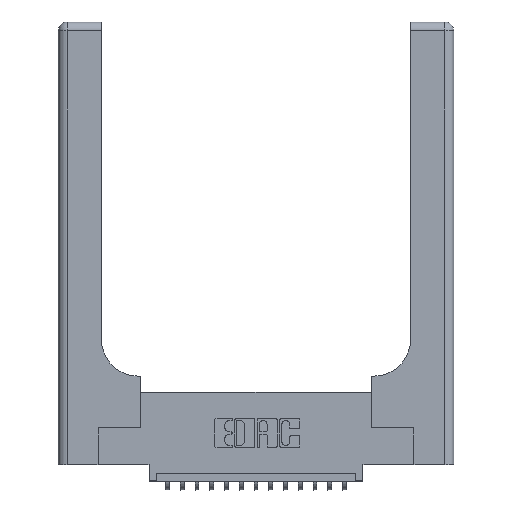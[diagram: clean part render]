
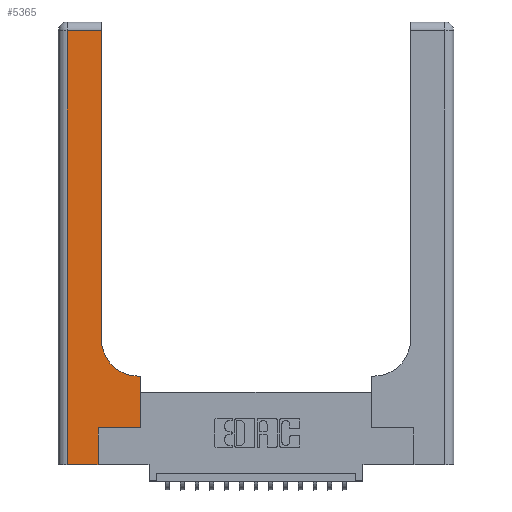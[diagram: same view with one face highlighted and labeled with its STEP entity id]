
A CAD part, top view. The second image highlights one B-rep face of the part: STEP entity #5365.
In plain terms, the highlighted planar face has unit normal (0, 0, 1).
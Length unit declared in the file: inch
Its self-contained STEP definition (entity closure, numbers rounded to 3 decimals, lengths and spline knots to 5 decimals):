
#322 = LINE ( 'NONE', #1450, #18718 ) ;
#375 = FACE_OUTER_BOUND ( 'NONE', #7149, .T. ) ;
#377 = CARTESIAN_POINT ( 'NONE',  ( 0.06, 2.94, 0.37 ) ) ;
#713 = CARTESIAN_POINT ( 'NONE',  ( 0., 2.94, 0.37 ) ) ;
#1450 = CARTESIAN_POINT ( 'NONE',  ( 0.5585, 0.25, 0.37 ) ) ;
#1487 = CARTESIAN_POINT ( 'NONE',  ( 0.5415, 0.85, 0.37 ) ) ;
#2405 = EDGE_CURVE ( 'NONE', #10606, #6755, #6256, .T. ) ;
#2713 = ORIENTED_EDGE ( 'NONE', *, *, #6560, .T. ) ;
#2805 = CARTESIAN_POINT ( 'NONE',  ( 0.269, 0.25, 0.37 ) ) ;
#3157 = CARTESIAN_POINT ( 'NONE',  ( 0.2915, 3., 0.37 ) ) ;
#3464 = CARTESIAN_POINT ( 'NONE',  ( 0.2915, 0.6, 0.37 ) ) ;
#3772 = EDGE_CURVE ( 'NONE', #4561, #6391, #17874, .T. ) ;
#3784 = ORIENTED_EDGE ( 'NONE', *, *, #3772, .T. ) ;
#4359 = CARTESIAN_POINT ( 'NONE',  ( 0., 0., 0.37 ) ) ;
#4384 = LINE ( 'NONE', #8307, #5082 ) ;
#4395 = AXIS2_PLACEMENT_3D ( 'NONE', #1487, #4442, #5828 ) ;
#4442 = DIRECTION ( 'NONE',  ( 0., 0., -1. ) ) ;
#4561 = VERTEX_POINT ( 'NONE', #8616 ) ;
#4680 = DIRECTION ( 'NONE',  ( 1., 0., 0. ) ) ;
#4895 = DIRECTION ( 'NONE',  ( 0., -1., 0. ) ) ;
#4956 = VERTEX_POINT ( 'NONE', #13395 ) ;
#5082 = VECTOR ( 'NONE', #11375, 39.37008 ) ;
#5114 = DIRECTION ( 'NONE',  ( -1., 0., 0. ) ) ;
#5365 = ADVANCED_FACE ( 'NONE', ( #375 ), #12111, .F. ) ;
#5442 = EDGE_CURVE ( 'NONE', #11132, #18178, #17842, .T. ) ;
#5612 = DIRECTION ( 'NONE',  ( 0., 1., 0. ) ) ;
#5828 = DIRECTION ( 'NONE',  ( 1., 0., 0. ) ) ;
#6236 = ORIENTED_EDGE ( 'NONE', *, *, #13190, .T. ) ;
#6256 = LINE ( 'NONE', #3464, #8334 ) ;
#6391 = VERTEX_POINT ( 'NONE', #9600 ) ;
#6426 = VECTOR ( 'NONE', #7838, 39.37008 ) ;
#6560 = EDGE_CURVE ( 'NONE', #4956, #10606, #322, .T. ) ;
#6755 = VERTEX_POINT ( 'NONE', #12718 ) ;
#7149 = EDGE_LOOP ( 'NONE', ( #3784, #6236, #11499, #14602, #11961, #16135, #2713, #11330, #9094 ) ) ;
#7528 = DIRECTION ( 'NONE',  ( -1., 0., 0. ) ) ;
#7838 = DIRECTION ( 'NONE',  ( 1., 0., 0. ) ) ;
#8307 = CARTESIAN_POINT ( 'NONE',  ( 0.269, 0., 0.37 ) ) ;
#8334 = VECTOR ( 'NONE', #16461, 39.37008 ) ;
#8616 = CARTESIAN_POINT ( 'NONE',  ( 0.2915, 0.85, 0.37 ) ) ;
#8687 = VECTOR ( 'NONE', #5114, 39.37008 ) ;
#8854 = EDGE_CURVE ( 'NONE', #6755, #4561, #9188, .T. ) ;
#8856 = CARTESIAN_POINT ( 'NONE',  ( 0.06, 0., 0.37 ) ) ;
#9094 = ORIENTED_EDGE ( 'NONE', *, *, #8854, .T. ) ;
#9162 = DIRECTION ( 'NONE',  ( 0., 0., -1. ) ) ;
#9188 = CIRCLE ( 'NONE', #4395, 0.25 ) ;
#9600 = CARTESIAN_POINT ( 'NONE',  ( 0.2915, 2.94, 0.37 ) ) ;
#10606 = VERTEX_POINT ( 'NONE', #16197 ) ;
#10868 = VERTEX_POINT ( 'NONE', #2805 ) ;
#11132 = VERTEX_POINT ( 'NONE', #377 ) ;
#11330 = ORIENTED_EDGE ( 'NONE', *, *, #2405, .T. ) ;
#11375 = DIRECTION ( 'NONE',  ( 0., 1., 0. ) ) ;
#11397 = EDGE_CURVE ( 'NONE', #17665, #10868, #4384, .T. ) ;
#11499 = ORIENTED_EDGE ( 'NONE', *, *, #5442, .T. ) ;
#11740 = DIRECTION ( 'NONE',  ( 0., 1., 0. ) ) ;
#11921 = EDGE_CURVE ( 'NONE', #10868, #4956, #14277, .T. ) ;
#11961 = ORIENTED_EDGE ( 'NONE', *, *, #11397, .T. ) ;
#11970 = CARTESIAN_POINT ( 'NONE',  ( 0., 3., 0.37 ) ) ;
#12111 = PLANE ( 'NONE',  #15451 ) ;
#12405 = LINE ( 'NONE', #4359, #18140 ) ;
#12718 = CARTESIAN_POINT ( 'NONE',  ( 0.5415, 0.6, 0.37 ) ) ;
#13190 = EDGE_CURVE ( 'NONE', #6391, #11132, #18850, .T. ) ;
#13395 = CARTESIAN_POINT ( 'NONE',  ( 0.5585, 0.25, 0.37 ) ) ;
#13796 = CARTESIAN_POINT ( 'NONE',  ( 0.06, 3., 0.37 ) ) ;
#13862 = EDGE_CURVE ( 'NONE', #18178, #17665, #12405, .T. ) ;
#13976 = VECTOR ( 'NONE', #11740, 39.37008 ) ;
#14277 = LINE ( 'NONE', #17978, #6426 ) ;
#14602 = ORIENTED_EDGE ( 'NONE', *, *, #13862, .T. ) ;
#15451 = AXIS2_PLACEMENT_3D ( 'NONE', #11970, #9162, #7528 ) ;
#16135 = ORIENTED_EDGE ( 'NONE', *, *, #11921, .T. ) ;
#16197 = CARTESIAN_POINT ( 'NONE',  ( 0.5585, 0.6, 0.37 ) ) ;
#16461 = DIRECTION ( 'NONE',  ( -1., 0., 0. ) ) ;
#16917 = VECTOR ( 'NONE', #4895, 39.37008 ) ;
#17665 = VERTEX_POINT ( 'NONE', #17895 ) ;
#17842 = LINE ( 'NONE', #13796, #16917 ) ;
#17874 = LINE ( 'NONE', #3157, #13976 ) ;
#17895 = CARTESIAN_POINT ( 'NONE',  ( 0.269, 0., 0.37 ) ) ;
#17978 = CARTESIAN_POINT ( 'NONE',  ( 0.269, 0.25, 0.37 ) ) ;
#18140 = VECTOR ( 'NONE', #4680, 39.37008 ) ;
#18178 = VERTEX_POINT ( 'NONE', #8856 ) ;
#18718 = VECTOR ( 'NONE', #5612, 39.37008 ) ;
#18850 = LINE ( 'NONE', #713, #8687 ) ;
